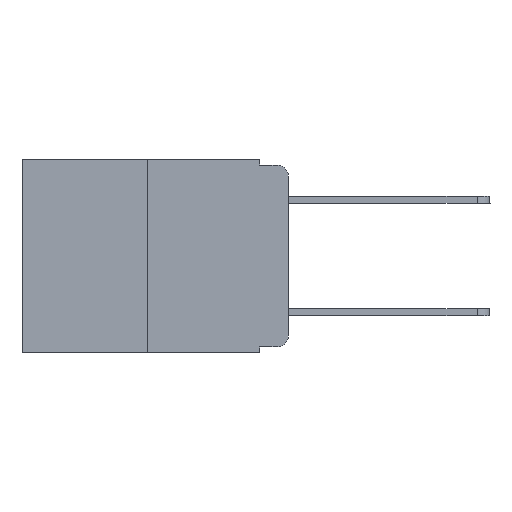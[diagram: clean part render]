
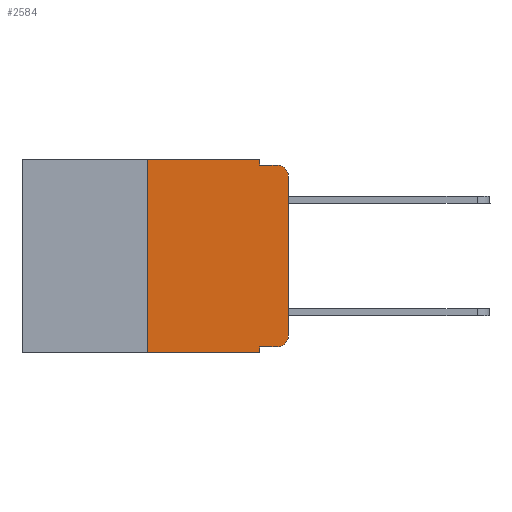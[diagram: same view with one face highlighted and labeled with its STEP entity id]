
A CAD part, left-side view. The second image highlights one B-rep face of the part: STEP entity #2584.
In plain terms, the highlighted planar face has unit normal (-1, 0, 0).
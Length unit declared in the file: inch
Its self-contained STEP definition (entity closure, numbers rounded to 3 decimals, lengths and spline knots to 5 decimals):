
#26 = LINE ( 'NONE', #6070, #5845 ) ;
#118 = AXIS2_PLACEMENT_3D ( 'NONE', #10357, #2552, #6046 ) ;
#234 = ORIENTED_EDGE ( 'NONE', *, *, #10940, .T. ) ;
#290 = ORIENTED_EDGE ( 'NONE', *, *, #5565, .F. ) ;
#376 = CIRCLE ( 'NONE', #1275, 0.02 ) ;
#424 = CARTESIAN_POINT ( 'NONE',  ( 0., 0.051, -0.343 ) ) ;
#536 = LINE ( 'NONE', #4131, #8849 ) ;
#672 = DIRECTION ( 'NONE',  ( 0., -1., 0. ) ) ;
#792 = EDGE_CURVE ( 'NONE', #8094, #6478, #536, .T. ) ;
#913 = LINE ( 'NONE', #3747, #10552 ) ;
#1060 = EDGE_LOOP ( 'NONE', ( #234, #1143, #6404, #1467, #11091, #2795, #9791, #290, #8416, #10124 ) ) ;
#1143 = ORIENTED_EDGE ( 'NONE', *, *, #3800, .T. ) ;
#1254 = VECTOR ( 'NONE', #7616, 39.37008 ) ;
#1275 = AXIS2_PLACEMENT_3D ( 'NONE', #2050, #4658, #10785 ) ;
#1362 = FACE_OUTER_BOUND ( 'NONE', #1060, .T. ) ;
#1367 = EDGE_CURVE ( 'NONE', #5021, #5899, #3230, .T. ) ;
#1467 = ORIENTED_EDGE ( 'NONE', *, *, #1518, .F. ) ;
#1518 = EDGE_CURVE ( 'NONE', #9787, #9093, #4812, .T. ) ;
#1768 = DIRECTION ( 'NONE',  ( 0., -1., 0. ) ) ;
#2050 = CARTESIAN_POINT ( 'NONE',  ( 0., 0.02, -0.03 ) ) ;
#2183 = EDGE_CURVE ( 'NONE', #5899, #6959, #7952, .T. ) ;
#2275 = CARTESIAN_POINT ( 'NONE',  ( 0., 0.473, 0. ) ) ;
#2517 = DIRECTION ( 'NONE',  ( 0., -1., 0. ) ) ;
#2552 = DIRECTION ( 'NONE',  ( -1., 0., 0. ) ) ;
#2553 = CARTESIAN_POINT ( 'NONE',  ( 0., 0.473, -0.343 ) ) ;
#2577 = VERTEX_POINT ( 'NONE', #4727 ) ;
#2584 = ADVANCED_FACE ( 'NONE', ( #1362 ), #10077, .F. ) ;
#2652 = LINE ( 'NONE', #9611, #4549 ) ;
#2711 = VECTOR ( 'NONE', #9085, 39.37008 ) ;
#2795 = ORIENTED_EDGE ( 'NONE', *, *, #792, .F. ) ;
#3122 = CARTESIAN_POINT ( 'NONE',  ( 0., 0.051, -0.333 ) ) ;
#3178 = DIRECTION ( 'NONE',  ( 0., 0., -1. ) ) ;
#3230 = LINE ( 'NONE', #3122, #1254 ) ;
#3350 = LINE ( 'NONE', #9504, #6323 ) ;
#3747 = CARTESIAN_POINT ( 'NONE',  ( 0., 0.051, -0.01 ) ) ;
#3800 = EDGE_CURVE ( 'NONE', #6248, #2577, #376, .T. ) ;
#4114 = CARTESIAN_POINT ( 'NONE',  ( 0., 0., -0.313 ) ) ;
#4131 = CARTESIAN_POINT ( 'NONE',  ( 0., 0.25, 0. ) ) ;
#4549 = VECTOR ( 'NONE', #10296, 39.37008 ) ;
#4658 = DIRECTION ( 'NONE',  ( -1., 0., 0. ) ) ;
#4727 = CARTESIAN_POINT ( 'NONE',  ( 0., 0.02, -0.01 ) ) ;
#4812 = LINE ( 'NONE', #6643, #2711 ) ;
#5021 = VERTEX_POINT ( 'NONE', #6967 ) ;
#5535 = CARTESIAN_POINT ( 'NONE',  ( 0., 0.051, -0.01 ) ) ;
#5565 = EDGE_CURVE ( 'NONE', #5021, #10098, #2652, .T. ) ;
#5689 = CARTESIAN_POINT ( 'NONE',  ( 0., 0.02, -0.333 ) ) ;
#5756 = DIRECTION ( 'NONE',  ( 1., 0., 0. ) ) ;
#5845 = VECTOR ( 'NONE', #2517, 39.37008 ) ;
#5899 = VERTEX_POINT ( 'NONE', #5689 ) ;
#5993 = CARTESIAN_POINT ( 'NONE',  ( 0., 0.25, -0.343 ) ) ;
#6046 = DIRECTION ( 'NONE',  ( 0., 0., -1. ) ) ;
#6070 = CARTESIAN_POINT ( 'NONE',  ( 0., 0.473, 0. ) ) ;
#6248 = VERTEX_POINT ( 'NONE', #10047 ) ;
#6323 = VECTOR ( 'NONE', #6896, 39.37008 ) ;
#6404 = ORIENTED_EDGE ( 'NONE', *, *, #8182, .F. ) ;
#6478 = VERTEX_POINT ( 'NONE', #8046 ) ;
#6643 = CARTESIAN_POINT ( 'NONE',  ( 0., 0.051, 0. ) ) ;
#6795 = CARTESIAN_POINT ( 'NONE',  ( 0., 0.051, 0. ) ) ;
#6896 = DIRECTION ( 'NONE',  ( 0., 0., 1. ) ) ;
#6959 = VERTEX_POINT ( 'NONE', #4114 ) ;
#6967 = CARTESIAN_POINT ( 'NONE',  ( 0., 0.051, -0.333 ) ) ;
#7616 = DIRECTION ( 'NONE',  ( 0., -1., 0. ) ) ;
#7952 = CIRCLE ( 'NONE', #118, 0.02 ) ;
#8046 = CARTESIAN_POINT ( 'NONE',  ( 0., 0.25, 0. ) ) ;
#8094 = VERTEX_POINT ( 'NONE', #5993 ) ;
#8182 = EDGE_CURVE ( 'NONE', #9093, #2577, #913, .T. ) ;
#8416 = ORIENTED_EDGE ( 'NONE', *, *, #1367, .T. ) ;
#8543 = LINE ( 'NONE', #2553, #9820 ) ;
#8849 = VECTOR ( 'NONE', #9191, 39.37008 ) ;
#8901 = EDGE_CURVE ( 'NONE', #6478, #9787, #26, .T. ) ;
#9085 = DIRECTION ( 'NONE',  ( 0., 0., -1. ) ) ;
#9093 = VERTEX_POINT ( 'NONE', #5535 ) ;
#9191 = DIRECTION ( 'NONE',  ( 0., 0., 1. ) ) ;
#9418 = AXIS2_PLACEMENT_3D ( 'NONE', #2275, #5756, #3178 ) ;
#9504 = CARTESIAN_POINT ( 'NONE',  ( 0., 0., 0. ) ) ;
#9611 = CARTESIAN_POINT ( 'NONE',  ( 0., 0.051, 0. ) ) ;
#9700 = EDGE_CURVE ( 'NONE', #8094, #10098, #8543, .T. ) ;
#9787 = VERTEX_POINT ( 'NONE', #6795 ) ;
#9791 = ORIENTED_EDGE ( 'NONE', *, *, #9700, .T. ) ;
#9820 = VECTOR ( 'NONE', #672, 39.37008 ) ;
#10047 = CARTESIAN_POINT ( 'NONE',  ( 0., 0., -0.03 ) ) ;
#10077 = PLANE ( 'NONE',  #9418 ) ;
#10098 = VERTEX_POINT ( 'NONE', #424 ) ;
#10124 = ORIENTED_EDGE ( 'NONE', *, *, #2183, .T. ) ;
#10296 = DIRECTION ( 'NONE',  ( 0., 0., -1. ) ) ;
#10357 = CARTESIAN_POINT ( 'NONE',  ( 0., 0.02, -0.313 ) ) ;
#10552 = VECTOR ( 'NONE', #1768, 39.37008 ) ;
#10785 = DIRECTION ( 'NONE',  ( 0., 0., -1. ) ) ;
#10940 = EDGE_CURVE ( 'NONE', #6959, #6248, #3350, .T. ) ;
#11091 = ORIENTED_EDGE ( 'NONE', *, *, #8901, .F. ) ;
